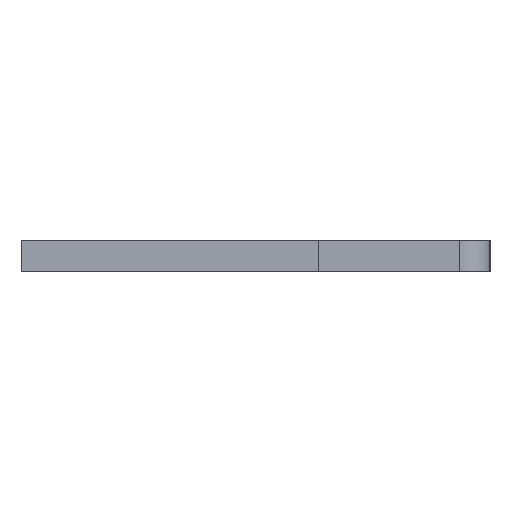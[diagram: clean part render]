
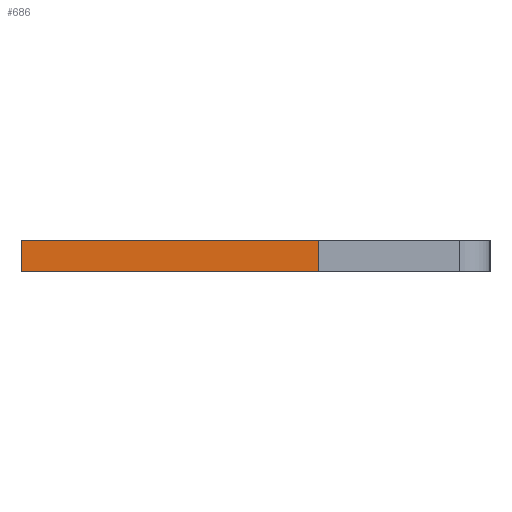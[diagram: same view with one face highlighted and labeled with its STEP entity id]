
A CAD part, left-side view. The second image highlights one B-rep face of the part: STEP entity #686.
In plain terms, the highlighted face is planar.
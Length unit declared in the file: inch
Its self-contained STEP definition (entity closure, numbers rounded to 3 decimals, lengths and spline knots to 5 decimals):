
#18 = VERTEX_POINT ( 'NONE', #1641 ) ;
#28 = CARTESIAN_POINT ( 'NONE',  ( 0.01, -0.04, -0.04 ) ) ;
#121 = ORIENTED_EDGE ( 'NONE', *, *, #433, .T. ) ;
#218 = LINE ( 'NONE', #407, #1823 ) ;
#325 = VERTEX_POINT ( 'NONE', #2357 ) ;
#337 = PLANE ( 'NONE',  #1367 ) ;
#407 = CARTESIAN_POINT ( 'NONE',  ( 0.01, 0.15, -0.04 ) ) ;
#433 = EDGE_CURVE ( 'NONE', #2061, #18, #1267, .T. ) ;
#471 = CARTESIAN_POINT ( 'NONE',  ( -0.01, -0.04, -0.04 ) ) ;
#501 = DIRECTION ( 'NONE',  ( -1., 0., 0. ) ) ;
#513 = DIRECTION ( 'NONE',  ( -1., 0., 0. ) ) ;
#675 = VECTOR ( 'NONE', #1458, 39.37008 ) ;
#686 = ADVANCED_FACE ( 'NONE', ( #2748 ), #337, .F. ) ;
#790 = CARTESIAN_POINT ( 'NONE',  ( 0.01, 0.15, -0.04 ) ) ;
#947 = CARTESIAN_POINT ( 'NONE',  ( 0.01, 0.15, -0.04 ) ) ;
#990 = LINE ( 'NONE', #28, #2711 ) ;
#1075 = EDGE_CURVE ( 'NONE', #325, #2163, #218, .T. ) ;
#1216 = CARTESIAN_POINT ( 'NONE',  ( -0.01, 0.15, -0.04 ) ) ;
#1242 = DIRECTION ( 'NONE',  ( 0., 0., 1. ) ) ;
#1267 = LINE ( 'NONE', #1216, #675 ) ;
#1367 = AXIS2_PLACEMENT_3D ( 'NONE', #790, #1242, #2817 ) ;
#1448 = VECTOR ( 'NONE', #513, 39.37008 ) ;
#1458 = DIRECTION ( 'NONE',  ( 0., 1., 0. ) ) ;
#1641 = CARTESIAN_POINT ( 'NONE',  ( -0.01, 0.15, -0.04 ) ) ;
#1721 = EDGE_LOOP ( 'NONE', ( #121, #1899, #2341, #1858 ) ) ;
#1823 = VECTOR ( 'NONE', #2648, 39.37008 ) ;
#1858 = ORIENTED_EDGE ( 'NONE', *, *, #1924, .T. ) ;
#1899 = ORIENTED_EDGE ( 'NONE', *, *, #2178, .F. ) ;
#1924 = EDGE_CURVE ( 'NONE', #325, #2061, #990, .T. ) ;
#2031 = LINE ( 'NONE', #947, #1448 ) ;
#2061 = VERTEX_POINT ( 'NONE', #471 ) ;
#2163 = VERTEX_POINT ( 'NONE', #2283 ) ;
#2178 = EDGE_CURVE ( 'NONE', #2163, #18, #2031, .T. ) ;
#2283 = CARTESIAN_POINT ( 'NONE',  ( 0.01, 0.15, -0.04 ) ) ;
#2341 = ORIENTED_EDGE ( 'NONE', *, *, #1075, .F. ) ;
#2357 = CARTESIAN_POINT ( 'NONE',  ( 0.01, -0.04, -0.04 ) ) ;
#2648 = DIRECTION ( 'NONE',  ( 0., 1., 0. ) ) ;
#2711 = VECTOR ( 'NONE', #501, 39.37008 ) ;
#2748 = FACE_OUTER_BOUND ( 'NONE', #1721, .T. ) ;
#2817 = DIRECTION ( 'NONE',  ( 1., 0., 0. ) ) ;
